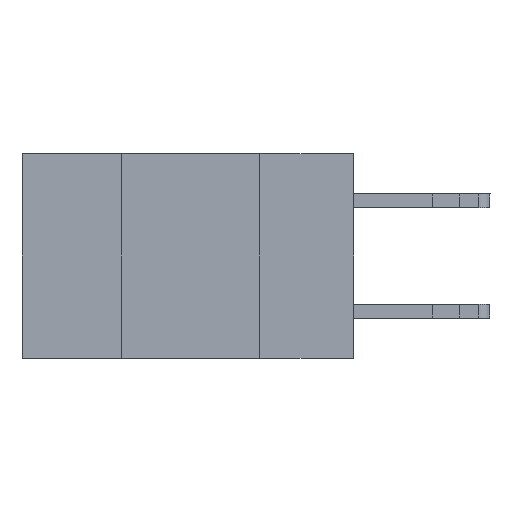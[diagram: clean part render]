
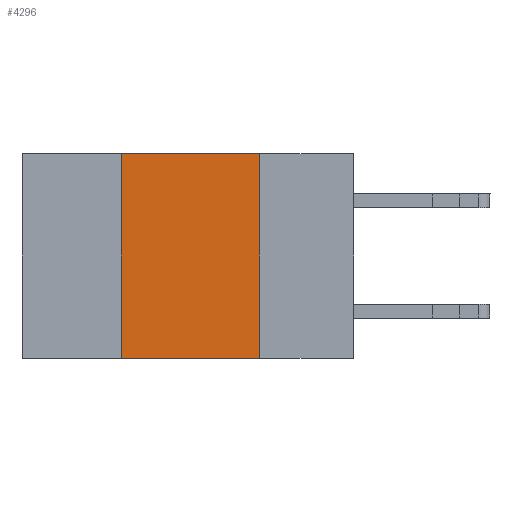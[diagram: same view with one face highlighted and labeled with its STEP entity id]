
A CAD part, left-side view. The second image highlights one B-rep face of the part: STEP entity #4296.
In plain terms, the highlighted planar face has unit normal (-1, 0, 0).
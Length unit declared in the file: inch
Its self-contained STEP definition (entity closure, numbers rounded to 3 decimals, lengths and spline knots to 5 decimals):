
#298 = CARTESIAN_POINT ( 'NONE',  ( 0., 0.6, -0.37 ) ) ;
#350 = CARTESIAN_POINT ( 'NONE',  ( 0., 0.17, 0. ) ) ;
#1124 = VERTEX_POINT ( 'NONE', #6300 ) ;
#1390 = ORIENTED_EDGE ( 'NONE', *, *, #11189, .T. ) ;
#1560 = ORIENTED_EDGE ( 'NONE', *, *, #13159, .F. ) ;
#2434 = CARTESIAN_POINT ( 'NONE',  ( 0., 0.6, 0. ) ) ;
#2891 = DIRECTION ( 'NONE',  ( 1., 0., 0. ) ) ;
#2910 = VECTOR ( 'NONE', #16456, 39.37008 ) ;
#3133 = DIRECTION ( 'NONE',  ( 0., -1., 0. ) ) ;
#3461 = EDGE_CURVE ( 'NONE', #13557, #15243, #14077, .T. ) ;
#4296 = ADVANCED_FACE ( 'NONE', ( #13843 ), #13268, .F. ) ;
#4374 = CARTESIAN_POINT ( 'NONE',  ( 0., 0.42, -0.37 ) ) ;
#4386 = DIRECTION ( 'NONE',  ( 0., 0., 1. ) ) ;
#4525 = LINE ( 'NONE', #2434, #14850 ) ;
#6088 = EDGE_CURVE ( 'NONE', #14683, #1124, #11526, .T. ) ;
#6300 = CARTESIAN_POINT ( 'NONE',  ( 0., 0.42, 0. ) ) ;
#6971 = DIRECTION ( 'NONE',  ( 0., 0., -1. ) ) ;
#7314 = AXIS2_PLACEMENT_3D ( 'NONE', #16218, #2891, #6971 ) ;
#8247 = EDGE_LOOP ( 'NONE', ( #16217, #1560, #11546, #1390 ) ) ;
#8251 = CARTESIAN_POINT ( 'NONE',  ( 0., 0.42, 0. ) ) ;
#9657 = VECTOR ( 'NONE', #3133, 39.37008 ) ;
#10655 = VECTOR ( 'NONE', #4386, 39.37008 ) ;
#11152 = CARTESIAN_POINT ( 'NONE',  ( 0., 0.17, 0. ) ) ;
#11189 = EDGE_CURVE ( 'NONE', #14683, #15243, #13228, .T. ) ;
#11526 = LINE ( 'NONE', #8251, #10655 ) ;
#11546 = ORIENTED_EDGE ( 'NONE', *, *, #6088, .F. ) ;
#11813 = DIRECTION ( 'NONE',  ( 0., -1., 0. ) ) ;
#13159 = EDGE_CURVE ( 'NONE', #1124, #13557, #4525, .T. ) ;
#13228 = LINE ( 'NONE', #298, #9657 ) ;
#13268 = PLANE ( 'NONE',  #7314 ) ;
#13557 = VERTEX_POINT ( 'NONE', #350 ) ;
#13843 = FACE_OUTER_BOUND ( 'NONE', #8247, .T. ) ;
#14077 = LINE ( 'NONE', #11152, #2910 ) ;
#14683 = VERTEX_POINT ( 'NONE', #4374 ) ;
#14849 = CARTESIAN_POINT ( 'NONE',  ( 0., 0.17, -0.37 ) ) ;
#14850 = VECTOR ( 'NONE', #11813, 39.37008 ) ;
#15243 = VERTEX_POINT ( 'NONE', #14849 ) ;
#16217 = ORIENTED_EDGE ( 'NONE', *, *, #3461, .F. ) ;
#16218 = CARTESIAN_POINT ( 'NONE',  ( 0., 0.6, 0. ) ) ;
#16456 = DIRECTION ( 'NONE',  ( 0., 0., -1. ) ) ;
